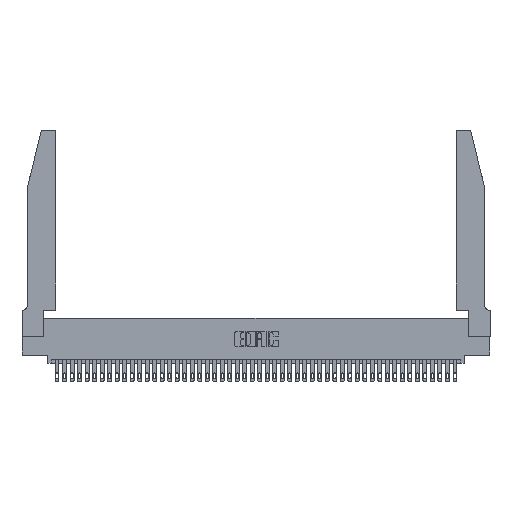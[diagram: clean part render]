
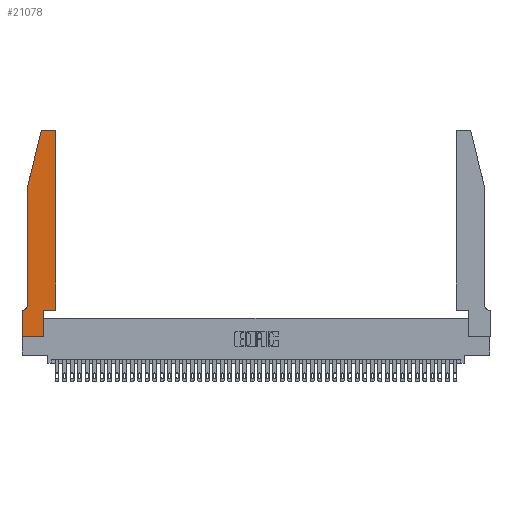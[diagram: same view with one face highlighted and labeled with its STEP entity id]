
A CAD part, top view. The second image highlights one B-rep face of the part: STEP entity #21078.
In plain terms, the highlighted planar face has unit normal (0, 0, 1).
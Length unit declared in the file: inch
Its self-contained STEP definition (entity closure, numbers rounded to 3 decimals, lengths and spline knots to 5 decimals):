
#123 = LINE ( 'NONE', #36838, #18849 ) ;
#353 = ORIENTED_EDGE ( 'NONE', *, *, #23281, .T. ) ;
#449 = VECTOR ( 'NONE', #37306, 39.37008 ) ;
#813 = VERTEX_POINT ( 'NONE', #32827 ) ;
#904 = ORIENTED_EDGE ( 'NONE', *, *, #11720, .T. ) ;
#1372 = VERTEX_POINT ( 'NONE', #2404 ) ;
#2262 = VERTEX_POINT ( 'NONE', #20029 ) ;
#2404 = CARTESIAN_POINT ( 'NONE',  ( 0.0755, 2., 0.37 ) ) ;
#2674 = DIRECTION ( 'NONE',  ( -1., 0., 0. ) ) ;
#2925 = CARTESIAN_POINT ( 'NONE',  ( 0.2865, 0., 0.37 ) ) ;
#2936 = CARTESIAN_POINT ( 'NONE',  ( 0.4505, 2.72, 0.37 ) ) ;
#4691 = DIRECTION ( 'NONE',  ( 0., 1., 0. ) ) ;
#5158 = DIRECTION ( 'NONE',  ( -1., 0., 0. ) ) ;
#5309 = DIRECTION ( 'NONE',  ( 1., 0., 0. ) ) ;
#5603 = ORIENTED_EDGE ( 'NONE', *, *, #39542, .T. ) ;
#6170 = ORIENTED_EDGE ( 'NONE', *, *, #10285, .T. ) ;
#6497 = CARTESIAN_POINT ( 'NONE',  ( 0.4505, 0.35, 0.37 ) ) ;
#6505 = CARTESIAN_POINT ( 'NONE',  ( 0.4205, 2.72, 0.37 ) ) ;
#6748 = AXIS2_PLACEMENT_3D ( 'NONE', #7633, #14569, #33044 ) ;
#6856 = CIRCLE ( 'NONE', #18950, 0.03 ) ;
#6887 = LINE ( 'NONE', #10506, #18464 ) ;
#7446 = FACE_OUTER_BOUND ( 'NONE', #17634, .T. ) ;
#7633 = CARTESIAN_POINT ( 'NONE',  ( 0., 0.35, 0.37 ) ) ;
#8369 = ORIENTED_EDGE ( 'NONE', *, *, #20510, .T. ) ;
#8942 = EDGE_CURVE ( 'NONE', #23217, #2262, #12335, .T. ) ;
#9009 = LINE ( 'NONE', #44591, #35991 ) ;
#10285 = EDGE_CURVE ( 'NONE', #1372, #14077, #123, .T. ) ;
#10477 = DIRECTION ( 'NONE',  ( 1., 0., 0. ) ) ;
#10506 = CARTESIAN_POINT ( 'NONE',  ( 0.2605, 2.75, 0.37 ) ) ;
#11720 = EDGE_CURVE ( 'NONE', #21155, #38927, #30873, .T. ) ;
#11777 = CARTESIAN_POINT ( 'NONE',  ( 0.2865, 0.35, 0.37 ) ) ;
#12335 = LINE ( 'NONE', #6497, #25036 ) ;
#12577 = VERTEX_POINT ( 'NONE', #2936 ) ;
#13524 = DIRECTION ( 'NONE',  ( -0.239, -0.971, 0. ) ) ;
#14077 = VERTEX_POINT ( 'NONE', #29272 ) ;
#14497 = VECTOR ( 'NONE', #4691, 39.37008 ) ;
#14569 = DIRECTION ( 'NONE',  ( 0., 0., 1. ) ) ;
#14636 = CARTESIAN_POINT ( 'NONE',  ( 0., 0., 0.37 ) ) ;
#16119 = EDGE_CURVE ( 'NONE', #38927, #23217, #26135, .T. ) ;
#16316 = LINE ( 'NONE', #42037, #36640 ) ;
#17048 = LINE ( 'NONE', #24921, #36236 ) ;
#17336 = DIRECTION ( 'NONE',  ( 0., 0., 1. ) ) ;
#17429 = DIRECTION ( 'NONE',  ( 0., -1., 0. ) ) ;
#17634 = EDGE_LOOP ( 'NONE', ( #353, #20788, #5603, #6170, #8369, #28957, #26706, #904, #34459, #35126, #45465, #19421 ) ) ;
#18464 = VECTOR ( 'NONE', #45359, 39.37008 ) ;
#18522 = CARTESIAN_POINT ( 'NONE',  ( 0.0055, 0.35, 0.37 ) ) ;
#18587 = VERTEX_POINT ( 'NONE', #43674 ) ;
#18849 = VECTOR ( 'NONE', #22844, 39.37008 ) ;
#18950 = AXIS2_PLACEMENT_3D ( 'NONE', #40905, #23377, #5309 ) ;
#19421 = ORIENTED_EDGE ( 'NONE', *, *, #43191, .T. ) ;
#19532 = CARTESIAN_POINT ( 'NONE',  ( 0.4505, 0.35, 0.37 ) ) ;
#19638 = VECTOR ( 'NONE', #26447, 39.37008 ) ;
#20029 = CARTESIAN_POINT ( 'NONE',  ( 0.4505, 0.35, 0.37 ) ) ;
#20510 = EDGE_CURVE ( 'NONE', #14077, #20609, #22418, .T. ) ;
#20609 = VERTEX_POINT ( 'NONE', #18522 ) ;
#20788 = ORIENTED_EDGE ( 'NONE', *, *, #40012, .T. ) ;
#20925 = EDGE_CURVE ( 'NONE', #2262, #12577, #38350, .T. ) ;
#21078 = ADVANCED_FACE ( 'NONE', ( #7446 ), #35681, .T. ) ;
#21155 = VERTEX_POINT ( 'NONE', #35745 ) ;
#21831 = CARTESIAN_POINT ( 'NONE',  ( 0.25487, 2.72718, 0.37 ) ) ;
#22418 = CIRCLE ( 'NONE', #27708, 0.07 ) ;
#22844 = DIRECTION ( 'NONE',  ( 0., -1., 0. ) ) ;
#23217 = VERTEX_POINT ( 'NONE', #26198 ) ;
#23281 = EDGE_CURVE ( 'NONE', #813, #38412, #6887, .T. ) ;
#23377 = DIRECTION ( 'NONE',  ( 0., 0., 1. ) ) ;
#24921 = CARTESIAN_POINT ( 'NONE',  ( 0., 0., 0.37 ) ) ;
#25036 = VECTOR ( 'NONE', #29720, 39.37008 ) ;
#25666 = CARTESIAN_POINT ( 'NONE',  ( 0.0055, 0.42, 0.37 ) ) ;
#26135 = LINE ( 'NONE', #11777, #14497 ) ;
#26198 = CARTESIAN_POINT ( 'NONE',  ( 0.2865, 0.35, 0.37 ) ) ;
#26447 = DIRECTION ( 'NONE',  ( 0., 1., 0. ) ) ;
#26646 = CIRCLE ( 'NONE', #37939, 0.03 ) ;
#26706 = ORIENTED_EDGE ( 'NONE', *, *, #27067, .T. ) ;
#27067 = EDGE_CURVE ( 'NONE', #18587, #21155, #17048, .T. ) ;
#27708 = AXIS2_PLACEMENT_3D ( 'NONE', #25666, #32882, #5158 ) ;
#28957 = ORIENTED_EDGE ( 'NONE', *, *, #40186, .T. ) ;
#29272 = CARTESIAN_POINT ( 'NONE',  ( 0.0755, 0.42, 0.37 ) ) ;
#29720 = DIRECTION ( 'NONE',  ( 1., 0., 0. ) ) ;
#30873 = LINE ( 'NONE', #14636, #449 ) ;
#32351 = CARTESIAN_POINT ( 'NONE',  ( 0.284, 2.75, 0.37 ) ) ;
#32827 = CARTESIAN_POINT ( 'NONE',  ( 0.4205, 2.75, 0.37 ) ) ;
#32882 = DIRECTION ( 'NONE',  ( 0., 0., -1. ) ) ;
#33044 = DIRECTION ( 'NONE',  ( 1., 0., 0. ) ) ;
#34459 = ORIENTED_EDGE ( 'NONE', *, *, #16119, .T. ) ;
#35126 = ORIENTED_EDGE ( 'NONE', *, *, #8942, .T. ) ;
#35681 = PLANE ( 'NONE',  #6748 ) ;
#35745 = CARTESIAN_POINT ( 'NONE',  ( 0., 0., 0.37 ) ) ;
#35991 = VECTOR ( 'NONE', #2674, 39.37008 ) ;
#36236 = VECTOR ( 'NONE', #17429, 39.37008 ) ;
#36640 = VECTOR ( 'NONE', #13524, 39.37008 ) ;
#36838 = CARTESIAN_POINT ( 'NONE',  ( 0.0755, 2., 0.37 ) ) ;
#37115 = VERTEX_POINT ( 'NONE', #21831 ) ;
#37306 = DIRECTION ( 'NONE',  ( 1., 0., 0. ) ) ;
#37939 = AXIS2_PLACEMENT_3D ( 'NONE', #6505, #17336, #10477 ) ;
#38350 = LINE ( 'NONE', #19532, #19638 ) ;
#38412 = VERTEX_POINT ( 'NONE', #32351 ) ;
#38927 = VERTEX_POINT ( 'NONE', #2925 ) ;
#39542 = EDGE_CURVE ( 'NONE', #37115, #1372, #16316, .T. ) ;
#40012 = EDGE_CURVE ( 'NONE', #38412, #37115, #6856, .T. ) ;
#40186 = EDGE_CURVE ( 'NONE', #20609, #18587, #9009, .T. ) ;
#40905 = CARTESIAN_POINT ( 'NONE',  ( 0.284, 2.72, 0.37 ) ) ;
#42037 = CARTESIAN_POINT ( 'NONE',  ( 0.0755, 2., 0.37 ) ) ;
#43191 = EDGE_CURVE ( 'NONE', #12577, #813, #26646, .T. ) ;
#43674 = CARTESIAN_POINT ( 'NONE',  ( 0., 0.35, 0.37 ) ) ;
#44591 = CARTESIAN_POINT ( 'NONE',  ( 0.0755, 0.35, 0.37 ) ) ;
#45359 = DIRECTION ( 'NONE',  ( -1., 0., 0. ) ) ;
#45465 = ORIENTED_EDGE ( 'NONE', *, *, #20925, .T. ) ;
